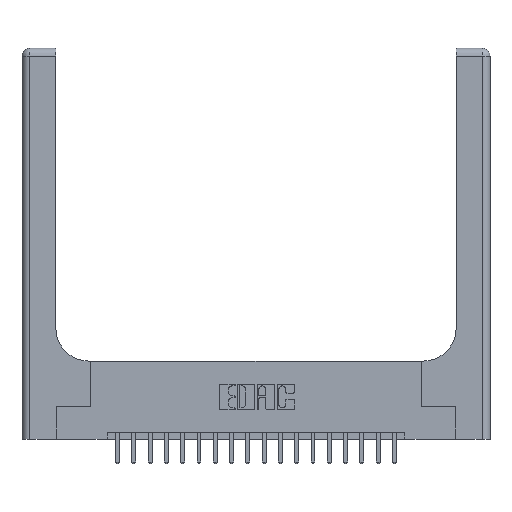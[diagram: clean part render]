
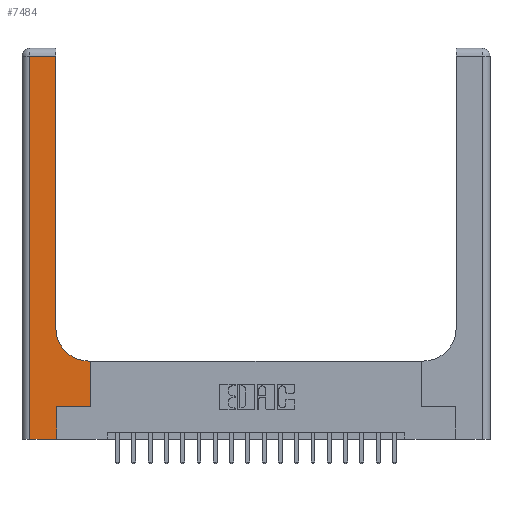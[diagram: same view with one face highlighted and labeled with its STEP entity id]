
A CAD part, top view. The second image highlights one B-rep face of the part: STEP entity #7484.
In plain terms, the highlighted planar face has unit normal (0, 0, 1).
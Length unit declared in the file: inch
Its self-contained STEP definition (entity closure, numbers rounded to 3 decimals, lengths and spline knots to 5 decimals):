
#330 = ORIENTED_EDGE ( 'NONE', *, *, #20457, .T. ) ;
#429 = DIRECTION ( 'NONE',  ( 0., 1., 0. ) ) ;
#513 = VECTOR ( 'NONE', #11240, 39.37008 ) ;
#534 = CARTESIAN_POINT ( 'NONE',  ( 0., 2.94, 0.37 ) ) ;
#1415 = ORIENTED_EDGE ( 'NONE', *, *, #17175, .T. ) ;
#1489 = CARTESIAN_POINT ( 'NONE',  ( 0.528, 0.25, 0.37 ) ) ;
#1493 = VERTEX_POINT ( 'NONE', #11243 ) ;
#1613 = EDGE_CURVE ( 'NONE', #6899, #6478, #4011, .T. ) ;
#1888 = CIRCLE ( 'NONE', #3926, 0.25 ) ;
#1994 = CARTESIAN_POINT ( 'NONE',  ( 0.26, 0.85, 0.37 ) ) ;
#2159 = EDGE_LOOP ( 'NONE', ( #14560, #13544, #18428, #330, #17842, #17520, #2551, #1415, #9579 ) ) ;
#2200 = CARTESIAN_POINT ( 'NONE',  ( 0.265, 0., 0.37 ) ) ;
#2551 = ORIENTED_EDGE ( 'NONE', *, *, #17722, .T. ) ;
#2678 = DIRECTION ( 'NONE',  ( 1., 0., 0. ) ) ;
#3891 = DIRECTION ( 'NONE',  ( 0., 1., 0. ) ) ;
#3926 = AXIS2_PLACEMENT_3D ( 'NONE', #17201, #14378, #9444 ) ;
#4011 = LINE ( 'NONE', #534, #19730 ) ;
#4257 = CARTESIAN_POINT ( 'NONE',  ( 0.265, 0.25, 0.37 ) ) ;
#4502 = CARTESIAN_POINT ( 'NONE',  ( 0.06, 2.94, 0.37 ) ) ;
#4785 = DIRECTION ( 'NONE',  ( -1., 0., 0. ) ) ;
#4847 = PLANE ( 'NONE',  #9859 ) ;
#5238 = VERTEX_POINT ( 'NONE', #15271 ) ;
#5979 = VECTOR ( 'NONE', #6475, 39.37008 ) ;
#6256 = LINE ( 'NONE', #18791, #9549 ) ;
#6475 = DIRECTION ( 'NONE',  ( 1., 0., 0. ) ) ;
#6478 = VERTEX_POINT ( 'NONE', #4502 ) ;
#6569 = VECTOR ( 'NONE', #429, 39.37008 ) ;
#6899 = VERTEX_POINT ( 'NONE', #7323 ) ;
#7084 = DIRECTION ( 'NONE',  ( 0., -1., 0. ) ) ;
#7094 = VERTEX_POINT ( 'NONE', #7157 ) ;
#7157 = CARTESIAN_POINT ( 'NONE',  ( 0.265, 0.25, 0.37 ) ) ;
#7323 = CARTESIAN_POINT ( 'NONE',  ( 0.26, 2.94, 0.37 ) ) ;
#7484 = ADVANCED_FACE ( 'NONE', ( #19174 ), #4847, .F. ) ;
#8801 = VERTEX_POINT ( 'NONE', #9576 ) ;
#9254 = LINE ( 'NONE', #1489, #513 ) ;
#9444 = DIRECTION ( 'NONE',  ( 1., 0., 0. ) ) ;
#9549 = VECTOR ( 'NONE', #4785, 39.37008 ) ;
#9576 = CARTESIAN_POINT ( 'NONE',  ( 0.528, 0.25, 0.37 ) ) ;
#9579 = ORIENTED_EDGE ( 'NONE', *, *, #19518, .T. ) ;
#9615 = CARTESIAN_POINT ( 'NONE',  ( 0.265, 0., 0.37 ) ) ;
#9859 = AXIS2_PLACEMENT_3D ( 'NONE', #19384, #14694, #11228 ) ;
#10647 = VERTEX_POINT ( 'NONE', #1994 ) ;
#11228 = DIRECTION ( 'NONE',  ( -1., 0., 0. ) ) ;
#11240 = DIRECTION ( 'NONE',  ( 0., 1., 0. ) ) ;
#11243 = CARTESIAN_POINT ( 'NONE',  ( 0.528, 0.6, 0.37 ) ) ;
#11708 = EDGE_CURVE ( 'NONE', #10647, #6899, #13029, .T. ) ;
#11805 = CARTESIAN_POINT ( 'NONE',  ( 0.06, 3., 0.37 ) ) ;
#12463 = VERTEX_POINT ( 'NONE', #9615 ) ;
#13029 = LINE ( 'NONE', #13346, #6569 ) ;
#13346 = CARTESIAN_POINT ( 'NONE',  ( 0.26, 3., 0.37 ) ) ;
#13544 = ORIENTED_EDGE ( 'NONE', *, *, #1613, .T. ) ;
#14373 = CARTESIAN_POINT ( 'NONE',  ( 0.06, 0., 0.37 ) ) ;
#14378 = DIRECTION ( 'NONE',  ( 0., 0., -1. ) ) ;
#14560 = ORIENTED_EDGE ( 'NONE', *, *, #11708, .T. ) ;
#14694 = DIRECTION ( 'NONE',  ( 0., 0., -1. ) ) ;
#15271 = CARTESIAN_POINT ( 'NONE',  ( 0.51, 0.6, 0.37 ) ) ;
#15278 = EDGE_CURVE ( 'NONE', #12463, #7094, #16987, .T. ) ;
#16138 = EDGE_CURVE ( 'NONE', #7094, #8801, #18490, .T. ) ;
#16916 = VECTOR ( 'NONE', #3891, 39.37008 ) ;
#16987 = LINE ( 'NONE', #2200, #16916 ) ;
#17175 = EDGE_CURVE ( 'NONE', #1493, #5238, #6256, .T. ) ;
#17201 = CARTESIAN_POINT ( 'NONE',  ( 0.51, 0.85, 0.37 ) ) ;
#17520 = ORIENTED_EDGE ( 'NONE', *, *, #16138, .T. ) ;
#17656 = VECTOR ( 'NONE', #7084, 39.37008 ) ;
#17722 = EDGE_CURVE ( 'NONE', #8801, #1493, #9254, .T. ) ;
#17842 = ORIENTED_EDGE ( 'NONE', *, *, #15278, .T. ) ;
#17910 = VECTOR ( 'NONE', #2678, 39.37008 ) ;
#18129 = VERTEX_POINT ( 'NONE', #14373 ) ;
#18371 = LINE ( 'NONE', #11805, #17656 ) ;
#18428 = ORIENTED_EDGE ( 'NONE', *, *, #20627, .T. ) ;
#18446 = DIRECTION ( 'NONE',  ( -1., 0., 0. ) ) ;
#18490 = LINE ( 'NONE', #4257, #17910 ) ;
#18791 = CARTESIAN_POINT ( 'NONE',  ( 0.26, 0.6, 0.37 ) ) ;
#19174 = FACE_OUTER_BOUND ( 'NONE', #2159, .T. ) ;
#19384 = CARTESIAN_POINT ( 'NONE',  ( 0., 3., 0.37 ) ) ;
#19428 = CARTESIAN_POINT ( 'NONE',  ( 0., 0., 0.37 ) ) ;
#19518 = EDGE_CURVE ( 'NONE', #5238, #10647, #1888, .T. ) ;
#19730 = VECTOR ( 'NONE', #18446, 39.37008 ) ;
#20457 = EDGE_CURVE ( 'NONE', #18129, #12463, #20713, .T. ) ;
#20627 = EDGE_CURVE ( 'NONE', #6478, #18129, #18371, .T. ) ;
#20713 = LINE ( 'NONE', #19428, #5979 ) ;
